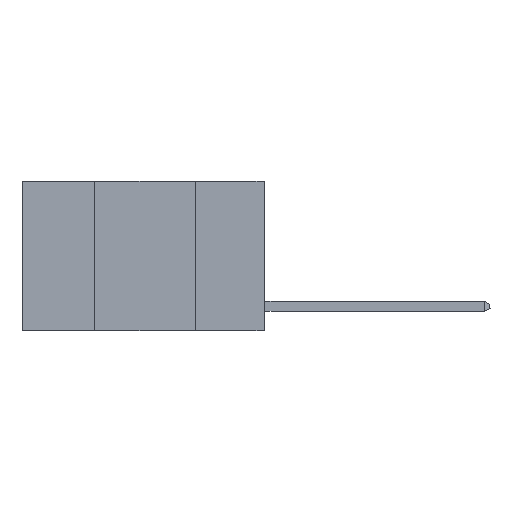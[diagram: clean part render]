
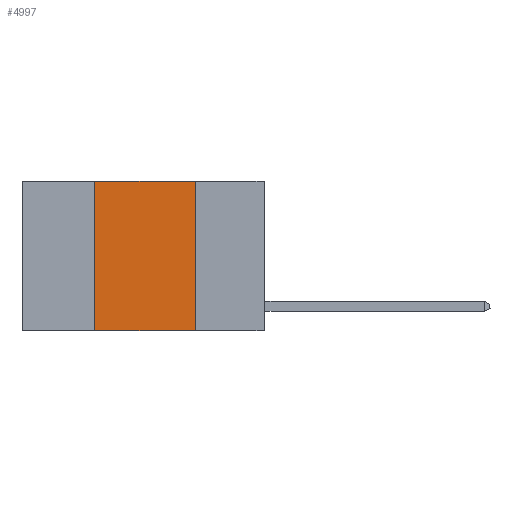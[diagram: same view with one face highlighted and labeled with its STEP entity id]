
A CAD part, left-side view. The second image highlights one B-rep face of the part: STEP entity #4997.
In plain terms, the highlighted planar face has unit normal (-1, 0, 0).
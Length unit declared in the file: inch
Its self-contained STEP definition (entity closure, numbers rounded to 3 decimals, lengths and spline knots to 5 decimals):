
#641 = LINE ( 'NONE', #7545, #2830 ) ;
#893 = CARTESIAN_POINT ( 'NONE',  ( 0., 0.42, 0. ) ) ;
#978 = ORIENTED_EDGE ( 'NONE', *, *, #4181, .F. ) ;
#1562 = AXIS2_PLACEMENT_3D ( 'NONE', #5607, #5666, #9718 ) ;
#1611 = FACE_OUTER_BOUND ( 'NONE', #11265, .T. ) ;
#1676 = PLANE ( 'NONE',  #1562 ) ;
#1740 = CARTESIAN_POINT ( 'NONE',  ( 0., 0.42, 0. ) ) ;
#1976 = CARTESIAN_POINT ( 'NONE',  ( 0., 0.17, 0. ) ) ;
#1983 = LINE ( 'NONE', #7830, #12069 ) ;
#2728 = LINE ( 'NONE', #1740, #8212 ) ;
#2818 = CARTESIAN_POINT ( 'NONE',  ( 0., 0.17, 0. ) ) ;
#2830 = VECTOR ( 'NONE', #3617, 39.37008 ) ;
#3228 = EDGE_CURVE ( 'NONE', #4565, #7254, #641, .T. ) ;
#3617 = DIRECTION ( 'NONE',  ( 0., -1., 0. ) ) ;
#3691 = ORIENTED_EDGE ( 'NONE', *, *, #6897, .F. ) ;
#4181 = EDGE_CURVE ( 'NONE', #10802, #6495, #1983, .T. ) ;
#4565 = VERTEX_POINT ( 'NONE', #10601 ) ;
#4997 = ADVANCED_FACE ( 'NONE', ( #1611 ), #1676, .F. ) ;
#5122 = DIRECTION ( 'NONE',  ( 0., 0., -1. ) ) ;
#5607 = CARTESIAN_POINT ( 'NONE',  ( 0., 0.6, 0. ) ) ;
#5666 = DIRECTION ( 'NONE',  ( 1., 0., 0. ) ) ;
#6495 = VERTEX_POINT ( 'NONE', #2818 ) ;
#6852 = DIRECTION ( 'NONE',  ( 0., 0., 1. ) ) ;
#6897 = EDGE_CURVE ( 'NONE', #4565, #10802, #2728, .T. ) ;
#7254 = VERTEX_POINT ( 'NONE', #8682 ) ;
#7355 = ORIENTED_EDGE ( 'NONE', *, *, #3228, .T. ) ;
#7443 = EDGE_CURVE ( 'NONE', #6495, #7254, #10273, .T. ) ;
#7545 = CARTESIAN_POINT ( 'NONE',  ( 0., 0.6, -0.37 ) ) ;
#7830 = CARTESIAN_POINT ( 'NONE',  ( 0., 0.6, 0. ) ) ;
#8212 = VECTOR ( 'NONE', #6852, 39.37008 ) ;
#8682 = CARTESIAN_POINT ( 'NONE',  ( 0., 0.17, -0.37 ) ) ;
#9718 = DIRECTION ( 'NONE',  ( 0., 0., -1. ) ) ;
#10224 = ORIENTED_EDGE ( 'NONE', *, *, #7443, .F. ) ;
#10273 = LINE ( 'NONE', #1976, #12801 ) ;
#10601 = CARTESIAN_POINT ( 'NONE',  ( 0., 0.42, -0.37 ) ) ;
#10802 = VERTEX_POINT ( 'NONE', #893 ) ;
#11265 = EDGE_LOOP ( 'NONE', ( #10224, #978, #3691, #7355 ) ) ;
#11894 = DIRECTION ( 'NONE',  ( 0., -1., 0. ) ) ;
#12069 = VECTOR ( 'NONE', #11894, 39.37008 ) ;
#12801 = VECTOR ( 'NONE', #5122, 39.37008 ) ;
